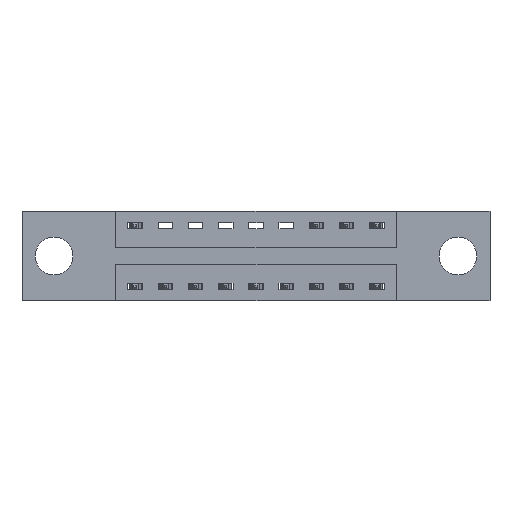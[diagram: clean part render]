
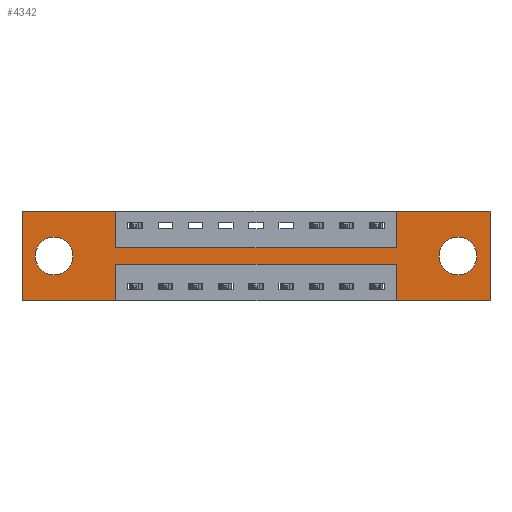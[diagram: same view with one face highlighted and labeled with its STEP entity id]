
A CAD part, front view. The second image highlights one B-rep face of the part: STEP entity #4342.
In plain terms, the highlighted planar face has unit normal (0, -1, 0).
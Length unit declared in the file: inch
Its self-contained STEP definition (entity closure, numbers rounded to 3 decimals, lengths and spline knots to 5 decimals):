
#171 = AXIS2_PLACEMENT_3D ( 'NONE', #2769, #8236, #3559 ) ;
#199 = VERTEX_POINT ( 'NONE', #3759 ) ;
#318 = CIRCLE ( 'NONE', #3553, 0.078 ) ;
#331 = DIRECTION ( 'NONE',  ( 0., 0., -1. ) ) ;
#591 = CARTESIAN_POINT ( 'NONE',  ( 0.3875, 0., -0.15 ) ) ;
#672 = CARTESIAN_POINT ( 'NONE',  ( 0., 0., 0. ) ) ;
#775 = DIRECTION ( 'NONE',  ( -1., 0., 0. ) ) ;
#853 = CARTESIAN_POINT ( 'NONE',  ( 0., 0., -0.37 ) ) ;
#1019 = CARTESIAN_POINT ( 'NONE',  ( 1.935, 0., 0. ) ) ;
#1076 = CARTESIAN_POINT ( 'NONE',  ( 0., 0., -0.37 ) ) ;
#1101 = ORIENTED_EDGE ( 'NONE', *, *, #5014, .F. ) ;
#1111 = CARTESIAN_POINT ( 'NONE',  ( 1.5475, 0., -0.37 ) ) ;
#1118 = EDGE_CURVE ( 'NONE', #2566, #4030, #4770, .T. ) ;
#1449 = VERTEX_POINT ( 'NONE', #5068 ) ;
#1493 = VECTOR ( 'NONE', #6222, 39.37008 ) ;
#1544 = CARTESIAN_POINT ( 'NONE',  ( 0., 0., 0. ) ) ;
#1707 = FACE_BOUND ( 'NONE', #8973, .T. ) ;
#1737 = ORIENTED_EDGE ( 'NONE', *, *, #2252, .T. ) ;
#1738 = EDGE_CURVE ( 'NONE', #5188, #2566, #9264, .T. ) ;
#1746 = DIRECTION ( 'NONE',  ( 0., 0., -1. ) ) ;
#1748 = ORIENTED_EDGE ( 'NONE', *, *, #6095, .T. ) ;
#1813 = VECTOR ( 'NONE', #8953, 39.37008 ) ;
#1815 = DIRECTION ( 'NONE',  ( 0., 0., -1. ) ) ;
#2074 = VECTOR ( 'NONE', #331, 39.37008 ) ;
#2097 = EDGE_CURVE ( 'NONE', #199, #9265, #9772, .T. ) ;
#2147 = CARTESIAN_POINT ( 'NONE',  ( 1.5475, 0., -0.37 ) ) ;
#2219 = EDGE_LOOP ( 'NONE', ( #1748, #8090 ) ) ;
#2252 = EDGE_CURVE ( 'NONE', #2328, #2808, #6190, .T. ) ;
#2268 = DIRECTION ( 'NONE',  ( 1., 0., 0. ) ) ;
#2307 = VECTOR ( 'NONE', #775, 39.37008 ) ;
#2328 = VERTEX_POINT ( 'NONE', #6135 ) ;
#2380 = DIRECTION ( 'NONE',  ( 1., 0., 0. ) ) ;
#2566 = VERTEX_POINT ( 'NONE', #7223 ) ;
#2655 = VERTEX_POINT ( 'NONE', #1076 ) ;
#2769 = CARTESIAN_POINT ( 'NONE',  ( 0.1325, 0., -0.185 ) ) ;
#2808 = VERTEX_POINT ( 'NONE', #2866 ) ;
#2866 = CARTESIAN_POINT ( 'NONE',  ( 0.1325, 0., -0.107 ) ) ;
#3032 = EDGE_CURVE ( 'NONE', #2655, #4207, #5673, .T. ) ;
#3091 = VECTOR ( 'NONE', #1746, 39.37008 ) ;
#3128 = ORIENTED_EDGE ( 'NONE', *, *, #3032, .F. ) ;
#3188 = LINE ( 'NONE', #6266, #5275 ) ;
#3194 = DIRECTION ( 'NONE',  ( 0., 1., 0. ) ) ;
#3305 = DIRECTION ( 'NONE',  ( 0., 0., 1. ) ) ;
#3424 = LINE ( 'NONE', #10080, #9183 ) ;
#3511 = DIRECTION ( 'NONE',  ( -1., 0., 0. ) ) ;
#3527 = VERTEX_POINT ( 'NONE', #2147 ) ;
#3553 = AXIS2_PLACEMENT_3D ( 'NONE', #7865, #3194, #8664 ) ;
#3559 = DIRECTION ( 'NONE',  ( 0., 0., 1. ) ) ;
#3646 = VECTOR ( 'NONE', #5986, 39.37008 ) ;
#3678 = DIRECTION ( 'NONE',  ( 0., 1., 0. ) ) ;
#3728 = EDGE_CURVE ( 'NONE', #4207, #5099, #3188, .T. ) ;
#3759 = CARTESIAN_POINT ( 'NONE',  ( 1.5475, 0., -0.22 ) ) ;
#3824 = DIRECTION ( 'NONE',  ( 1., 0., 0. ) ) ;
#3913 = LINE ( 'NONE', #5052, #2074 ) ;
#4030 = VERTEX_POINT ( 'NONE', #6582 ) ;
#4038 = DIRECTION ( 'NONE',  ( 0., 0., -1. ) ) ;
#4207 = VERTEX_POINT ( 'NONE', #672 ) ;
#4212 = EDGE_CURVE ( 'NONE', #6371, #6898, #3424, .T. ) ;
#4247 = CARTESIAN_POINT ( 'NONE',  ( 1.8025, 0., -0.185 ) ) ;
#4342 = ADVANCED_FACE ( 'NONE', ( #5880, #1707, #9807 ), #7908, .T. ) ;
#4411 = EDGE_CURVE ( 'NONE', #6898, #5188, #6952, .T. ) ;
#4496 = VERTEX_POINT ( 'NONE', #5777 ) ;
#4537 = EDGE_CURVE ( 'NONE', #5099, #6371, #3913, .T. ) ;
#4666 = ORIENTED_EDGE ( 'NONE', *, *, #1738, .F. ) ;
#4752 = ORIENTED_EDGE ( 'NONE', *, *, #4411, .F. ) ;
#4770 = LINE ( 'NONE', #1019, #8668 ) ;
#4820 = ORIENTED_EDGE ( 'NONE', *, *, #1118, .F. ) ;
#4861 = ORIENTED_EDGE ( 'NONE', *, *, #9610, .F. ) ;
#4874 = ORIENTED_EDGE ( 'NONE', *, *, #6139, .F. ) ;
#4903 = VECTOR ( 'NONE', #3305, 39.37008 ) ;
#4925 = ORIENTED_EDGE ( 'NONE', *, *, #2097, .F. ) ;
#4964 = ORIENTED_EDGE ( 'NONE', *, *, #4212, .F. ) ;
#4991 = ORIENTED_EDGE ( 'NONE', *, *, #6225, .T. ) ;
#5001 = CIRCLE ( 'NONE', #171, 0.078 ) ;
#5013 = DIRECTION ( 'NONE',  ( 0., 0., -1. ) ) ;
#5014 = EDGE_CURVE ( 'NONE', #1449, #2655, #9909, .T. ) ;
#5052 = CARTESIAN_POINT ( 'NONE',  ( 0.3875, 0., 0. ) ) ;
#5068 = CARTESIAN_POINT ( 'NONE',  ( 0.3875, 0., -0.37 ) ) ;
#5099 = VERTEX_POINT ( 'NONE', #7634 ) ;
#5188 = VERTEX_POINT ( 'NONE', #7731 ) ;
#5202 = CARTESIAN_POINT ( 'NONE',  ( 0., 0., -0.37 ) ) ;
#5275 = VECTOR ( 'NONE', #2380, 39.37008 ) ;
#5360 = VECTOR ( 'NONE', #3824, 39.37008 ) ;
#5673 = LINE ( 'NONE', #1544, #1493 ) ;
#5777 = CARTESIAN_POINT ( 'NONE',  ( 1.8025, 0., -0.263 ) ) ;
#5880 = FACE_BOUND ( 'NONE', #2219, .T. ) ;
#5889 = EDGE_CURVE ( 'NONE', #4496, #7745, #318, .T. ) ;
#5926 = LINE ( 'NONE', #7995, #3091 ) ;
#5986 = DIRECTION ( 'NONE',  ( -1., 0., 0. ) ) ;
#6095 = EDGE_CURVE ( 'NONE', #7745, #4496, #8047, .T. ) ;
#6135 = CARTESIAN_POINT ( 'NONE',  ( 0.1325, 0., -0.263 ) ) ;
#6139 = EDGE_CURVE ( 'NONE', #3527, #199, #7787, .T. ) ;
#6163 = AXIS2_PLACEMENT_3D ( 'NONE', #4247, #9704, #5013 ) ;
#6190 = CIRCLE ( 'NONE', #9232, 0.078 ) ;
#6222 = DIRECTION ( 'NONE',  ( 0., 0., 1. ) ) ;
#6225 = EDGE_CURVE ( 'NONE', #2808, #2328, #5001, .T. ) ;
#6266 = CARTESIAN_POINT ( 'NONE',  ( 0., 0., 0. ) ) ;
#6366 = EDGE_LOOP ( 'NONE', ( #8048, #4925, #4874, #4861, #4820, #4666, #4752, #4964, #7709, #7971, #3128, #1101 ) ) ;
#6371 = VERTEX_POINT ( 'NONE', #591 ) ;
#6582 = CARTESIAN_POINT ( 'NONE',  ( 1.935, 0., -0.37 ) ) ;
#6715 = LINE ( 'NONE', #10175, #2307 ) ;
#6898 = VERTEX_POINT ( 'NONE', #8430 ) ;
#6952 = LINE ( 'NONE', #9564, #4903 ) ;
#7044 = CARTESIAN_POINT ( 'NONE',  ( 1.8025, 0., -0.107 ) ) ;
#7223 = CARTESIAN_POINT ( 'NONE',  ( 1.935, 0., 0. ) ) ;
#7392 = CARTESIAN_POINT ( 'NONE',  ( 0.3875, 0., -0.22 ) ) ;
#7634 = CARTESIAN_POINT ( 'NONE',  ( 0.3875, 0., 0. ) ) ;
#7708 = CARTESIAN_POINT ( 'NONE',  ( 0., 0., 0. ) ) ;
#7709 = ORIENTED_EDGE ( 'NONE', *, *, #4537, .F. ) ;
#7731 = CARTESIAN_POINT ( 'NONE',  ( 1.5475, 0., 0. ) ) ;
#7745 = VERTEX_POINT ( 'NONE', #7044 ) ;
#7787 = LINE ( 'NONE', #1111, #1813 ) ;
#7865 = CARTESIAN_POINT ( 'NONE',  ( 1.8025, 0., -0.185 ) ) ;
#7906 = VECTOR ( 'NONE', #3511, 39.37008 ) ;
#7908 = PLANE ( 'NONE',  #8931 ) ;
#7971 = ORIENTED_EDGE ( 'NONE', *, *, #3728, .F. ) ;
#7995 = CARTESIAN_POINT ( 'NONE',  ( 0.3875, 0., -0.37 ) ) ;
#8047 = CIRCLE ( 'NONE', #6163, 0.078 ) ;
#8048 = ORIENTED_EDGE ( 'NONE', *, *, #8422, .F. ) ;
#8090 = ORIENTED_EDGE ( 'NONE', *, *, #5889, .T. ) ;
#8191 = CARTESIAN_POINT ( 'NONE',  ( 0.3875, 0., -0.22 ) ) ;
#8236 = DIRECTION ( 'NONE',  ( 0., 1., 0. ) ) ;
#8351 = CARTESIAN_POINT ( 'NONE',  ( 0.1325, 0., -0.185 ) ) ;
#8422 = EDGE_CURVE ( 'NONE', #9265, #1449, #5926, .T. ) ;
#8430 = CARTESIAN_POINT ( 'NONE',  ( 1.5475, 0., -0.15 ) ) ;
#8664 = DIRECTION ( 'NONE',  ( 0., 0., -1. ) ) ;
#8668 = VECTOR ( 'NONE', #1815, 39.37008 ) ;
#8704 = DIRECTION ( 'NONE',  ( 0., -1., 0. ) ) ;
#8931 = AXIS2_PLACEMENT_3D ( 'NONE', #853, #8704, #4038 ) ;
#8953 = DIRECTION ( 'NONE',  ( 0., 0., 1. ) ) ;
#8973 = EDGE_LOOP ( 'NONE', ( #4991, #1737 ) ) ;
#9159 = DIRECTION ( 'NONE',  ( 0., 0., 1. ) ) ;
#9183 = VECTOR ( 'NONE', #2268, 39.37008 ) ;
#9232 = AXIS2_PLACEMENT_3D ( 'NONE', #8351, #3678, #9159 ) ;
#9264 = LINE ( 'NONE', #7708, #5360 ) ;
#9265 = VERTEX_POINT ( 'NONE', #7392 ) ;
#9564 = CARTESIAN_POINT ( 'NONE',  ( 1.5475, 0., 0. ) ) ;
#9610 = EDGE_CURVE ( 'NONE', #4030, #3527, #6715, .T. ) ;
#9704 = DIRECTION ( 'NONE',  ( 0., 1., 0. ) ) ;
#9772 = LINE ( 'NONE', #8191, #7906 ) ;
#9807 = FACE_OUTER_BOUND ( 'NONE', #6366, .T. ) ;
#9909 = LINE ( 'NONE', #5202, #3646 ) ;
#10080 = CARTESIAN_POINT ( 'NONE',  ( 0.3875, 0., -0.15 ) ) ;
#10175 = CARTESIAN_POINT ( 'NONE',  ( 0., 0., -0.37 ) ) ;
